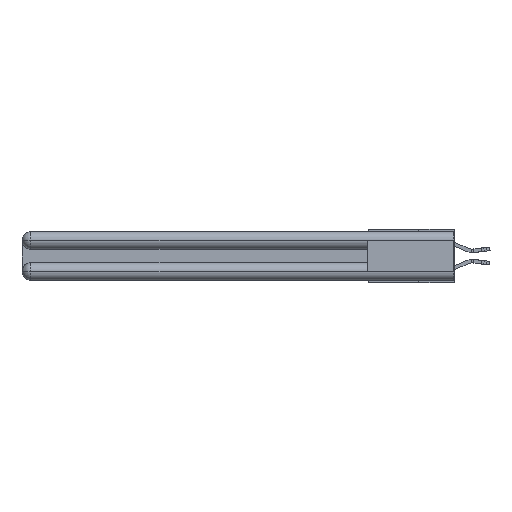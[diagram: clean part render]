
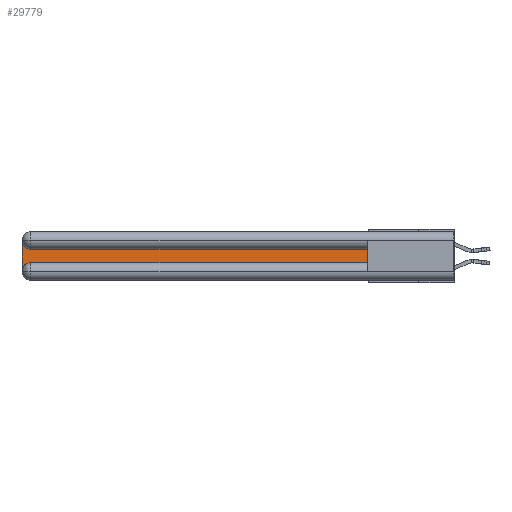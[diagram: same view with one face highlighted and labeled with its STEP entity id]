
A CAD part, left-side view. The second image highlights one B-rep face of the part: STEP entity #29779.
In plain terms, the highlighted planar face has unit normal (-1, 0, 0).
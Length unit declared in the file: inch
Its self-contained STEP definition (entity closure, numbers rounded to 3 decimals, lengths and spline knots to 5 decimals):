
#134 = EDGE_CURVE ( 'NONE', #25713, #24967, #32524, .T. ) ;
#494 = ORIENTED_EDGE ( 'NONE', *, *, #12896, .T. ) ;
#540 = CARTESIAN_POINT ( 'NONE',  ( 0.075, 2.94, -0.0625 ) ) ;
#1074 = EDGE_CURVE ( 'NONE', #8794, #8695, #11741, .T. ) ;
#1321 = ORIENTED_EDGE ( 'NONE', *, *, #1074, .T. ) ;
#1358 = CARTESIAN_POINT ( 'NONE',  ( 0.075, 0.6, -0.1225 ) ) ;
#2309 = VERTEX_POINT ( 'NONE', #6842 ) ;
#2972 = ORIENTED_EDGE ( 'NONE', *, *, #22345, .T. ) ;
#3096 = VECTOR ( 'NONE', #27744, 39.37008 ) ;
#3680 = EDGE_CURVE ( 'NONE', #8695, #28464, #31450, .T. ) ;
#3952 = CARTESIAN_POINT ( 'NONE',  ( 0.075, 2.94, -0.2775 ) ) ;
#5310 = DIRECTION ( 'NONE',  ( 0., -1., 0. ) ) ;
#5922 = VECTOR ( 'NONE', #5310, 39.37008 ) ;
#6461 = AXIS2_PLACEMENT_3D ( 'NONE', #16653, #24049, #29595 ) ;
#6524 = DIRECTION ( 'NONE',  ( 0., 0., -1. ) ) ;
#6842 = CARTESIAN_POINT ( 'NONE',  ( 0.075, 0.6, -0.2175 ) ) ;
#7167 = AXIS2_PLACEMENT_3D ( 'NONE', #540, #26694, #23916 ) ;
#8695 = VERTEX_POINT ( 'NONE', #12658 ) ;
#8794 = VERTEX_POINT ( 'NONE', #24953 ) ;
#10927 = LINE ( 'NONE', #29616, #5922 ) ;
#11741 = LINE ( 'NONE', #16405, #19621 ) ;
#12658 = CARTESIAN_POINT ( 'NONE',  ( 0.075, 3., -0.2775 ) ) ;
#12896 = EDGE_CURVE ( 'NONE', #24967, #8794, #13601, .T. ) ;
#13441 = CARTESIAN_POINT ( 'NONE',  ( 0.075, 0.6, -0.2175 ) ) ;
#13601 = CIRCLE ( 'NONE', #7167, 0.06 ) ;
#14049 = CARTESIAN_POINT ( 'NONE',  ( 0.075, 2.94, -0.1225 ) ) ;
#14249 = EDGE_CURVE ( 'NONE', #2309, #25713, #20140, .T. ) ;
#15423 = FACE_OUTER_BOUND ( 'NONE', #24371, .T. ) ;
#16405 = CARTESIAN_POINT ( 'NONE',  ( 0.075, 3., -0.2175 ) ) ;
#16653 = CARTESIAN_POINT ( 'NONE',  ( 0.075, 3., -0.1225 ) ) ;
#19621 = VECTOR ( 'NONE', #27460, 39.37008 ) ;
#20140 = LINE ( 'NONE', #13441, #32550 ) ;
#20217 = ORIENTED_EDGE ( 'NONE', *, *, #14249, .T. ) ;
#22345 = EDGE_CURVE ( 'NONE', #28464, #2309, #10927, .T. ) ;
#23916 = DIRECTION ( 'NONE',  ( 0., 0., -1. ) ) ;
#24028 = ORIENTED_EDGE ( 'NONE', *, *, #134, .T. ) ;
#24049 = DIRECTION ( 'NONE',  ( 1., 0., 0. ) ) ;
#24371 = EDGE_LOOP ( 'NONE', ( #24028, #494, #1321, #30941, #2972, #20217 ) ) ;
#24953 = CARTESIAN_POINT ( 'NONE',  ( 0.075, 3., -0.0625 ) ) ;
#24967 = VERTEX_POINT ( 'NONE', #14049 ) ;
#25713 = VERTEX_POINT ( 'NONE', #27770 ) ;
#26663 = CARTESIAN_POINT ( 'NONE',  ( 0.075, 2.94, -0.2175 ) ) ;
#26694 = DIRECTION ( 'NONE',  ( 1., 0., 0. ) ) ;
#26810 = PLANE ( 'NONE',  #6461 ) ;
#27460 = DIRECTION ( 'NONE',  ( 0., 0., -1. ) ) ;
#27685 = DIRECTION ( 'NONE',  ( 1., 0., 0. ) ) ;
#27744 = DIRECTION ( 'NONE',  ( 0., 1., 0. ) ) ;
#27770 = CARTESIAN_POINT ( 'NONE',  ( 0.075, 0.6, -0.1225 ) ) ;
#28464 = VERTEX_POINT ( 'NONE', #26663 ) ;
#29595 = DIRECTION ( 'NONE',  ( 0., 0., -1. ) ) ;
#29616 = CARTESIAN_POINT ( 'NONE',  ( 0.075, 0.6, -0.2175 ) ) ;
#29779 = ADVANCED_FACE ( 'NONE', ( #15423 ), #26810, .F. ) ;
#30941 = ORIENTED_EDGE ( 'NONE', *, *, #3680, .T. ) ;
#30965 = AXIS2_PLACEMENT_3D ( 'NONE', #3952, #27685, #6524 ) ;
#31450 = CIRCLE ( 'NONE', #30965, 0.06 ) ;
#31617 = DIRECTION ( 'NONE',  ( 0., 0., 1. ) ) ;
#32524 = LINE ( 'NONE', #1358, #3096 ) ;
#32550 = VECTOR ( 'NONE', #31617, 39.37008 ) ;
